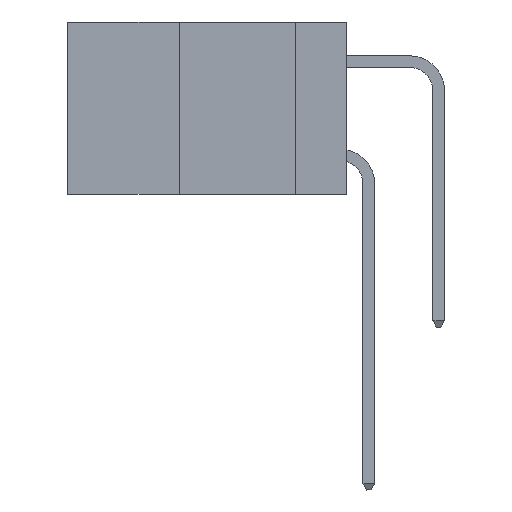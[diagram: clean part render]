
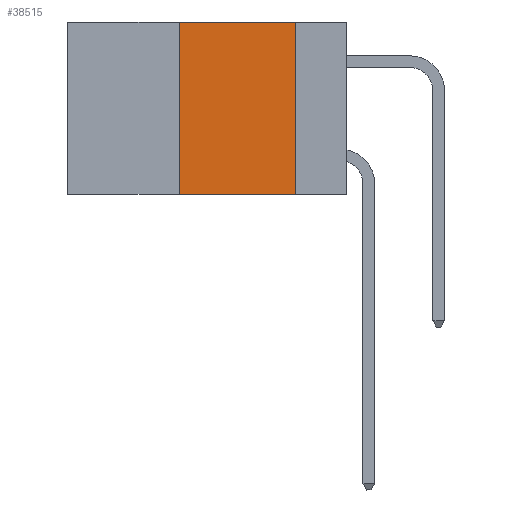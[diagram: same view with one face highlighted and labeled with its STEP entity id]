
A CAD part, left-side view. The second image highlights one B-rep face of the part: STEP entity #38515.
In plain terms, the highlighted planar face has unit normal (-1, 0, 0).
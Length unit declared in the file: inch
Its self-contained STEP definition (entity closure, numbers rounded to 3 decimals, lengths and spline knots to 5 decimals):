
#696 = EDGE_CURVE ( 'NONE', #6331, #9090, #6532, .T. ) ;
#933 = VECTOR ( 'NONE', #26438, 39.37008 ) ;
#1894 = LINE ( 'NONE', #14540, #29923 ) ;
#2241 = PLANE ( 'NONE',  #12782 ) ;
#4846 = DIRECTION ( 'NONE',  ( 1., 0., 0. ) ) ;
#5374 = FACE_OUTER_BOUND ( 'NONE', #17340, .T. ) ;
#6331 = VERTEX_POINT ( 'NONE', #34620 ) ;
#6532 = LINE ( 'NONE', #19927, #27312 ) ;
#7588 = ORIENTED_EDGE ( 'NONE', *, *, #696, .F. ) ;
#7923 = CARTESIAN_POINT ( 'NONE',  ( 0., 0.6, 0. ) ) ;
#9090 = VERTEX_POINT ( 'NONE', #12846 ) ;
#12782 = AXIS2_PLACEMENT_3D ( 'NONE', #7923, #4846, #29660 ) ;
#12846 = CARTESIAN_POINT ( 'NONE',  ( 0., 0.11, 0. ) ) ;
#14250 = ORIENTED_EDGE ( 'NONE', *, *, #29039, .F. ) ;
#14540 = CARTESIAN_POINT ( 'NONE',  ( 0., 0.36, 0. ) ) ;
#16633 = EDGE_CURVE ( 'NONE', #38703, #31801, #37752, .T. ) ;
#17132 = CARTESIAN_POINT ( 'NONE',  ( 0., 0.11, 0. ) ) ;
#17340 = EDGE_LOOP ( 'NONE', ( #14250, #7588, #39161, #39826 ) ) ;
#17812 = EDGE_CURVE ( 'NONE', #38703, #6331, #1894, .T. ) ;
#18423 = DIRECTION ( 'NONE',  ( 0., -1., 0. ) ) ;
#19927 = CARTESIAN_POINT ( 'NONE',  ( 0., 0.6, 0. ) ) ;
#22674 = LINE ( 'NONE', #17132, #933 ) ;
#23738 = VECTOR ( 'NONE', #18423, 39.37008 ) ;
#25220 = CARTESIAN_POINT ( 'NONE',  ( 0., 0.11, -0.37 ) ) ;
#26438 = DIRECTION ( 'NONE',  ( 0., 0., -1. ) ) ;
#27312 = VECTOR ( 'NONE', #28954, 39.37008 ) ;
#27845 = CARTESIAN_POINT ( 'NONE',  ( 0., 0.6, -0.37 ) ) ;
#28954 = DIRECTION ( 'NONE',  ( 0., -1., 0. ) ) ;
#29039 = EDGE_CURVE ( 'NONE', #9090, #31801, #22674, .T. ) ;
#29660 = DIRECTION ( 'NONE',  ( 0., 0., -1. ) ) ;
#29923 = VECTOR ( 'NONE', #32791, 39.37008 ) ;
#30198 = CARTESIAN_POINT ( 'NONE',  ( 0., 0.36, -0.37 ) ) ;
#31801 = VERTEX_POINT ( 'NONE', #25220 ) ;
#32791 = DIRECTION ( 'NONE',  ( 0., 0., 1. ) ) ;
#34620 = CARTESIAN_POINT ( 'NONE',  ( 0., 0.36, 0. ) ) ;
#37752 = LINE ( 'NONE', #27845, #23738 ) ;
#38515 = ADVANCED_FACE ( 'NONE', ( #5374 ), #2241, .F. ) ;
#38703 = VERTEX_POINT ( 'NONE', #30198 ) ;
#39161 = ORIENTED_EDGE ( 'NONE', *, *, #17812, .F. ) ;
#39826 = ORIENTED_EDGE ( 'NONE', *, *, #16633, .T. ) ;
